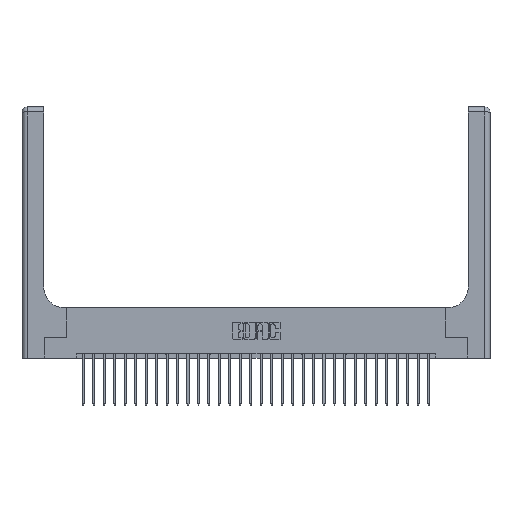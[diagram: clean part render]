
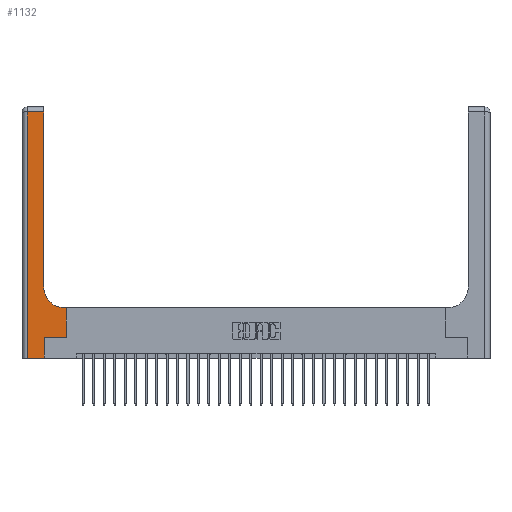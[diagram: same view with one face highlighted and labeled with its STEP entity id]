
A CAD part, top view. The second image highlights one B-rep face of the part: STEP entity #1132.
In plain terms, the highlighted planar face has unit normal (0, 0, 1).
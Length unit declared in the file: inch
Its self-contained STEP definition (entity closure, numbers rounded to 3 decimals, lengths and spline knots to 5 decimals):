
#255 = CARTESIAN_POINT ( 'NONE',  ( 0., 2.94, 0.37 ) ) ;
#324 = VERTEX_POINT ( 'NONE', #21119 ) ;
#370 = EDGE_CURVE ( 'NONE', #13079, #14114, #17188, .T. ) ;
#445 = CARTESIAN_POINT ( 'NONE',  ( 0.06, 2.94, 0.37 ) ) ;
#696 = DIRECTION ( 'NONE',  ( 1., 0., 0. ) ) ;
#823 = VECTOR ( 'NONE', #24106, 39.37008 ) ;
#900 = CARTESIAN_POINT ( 'NONE',  ( 0.51, 0.6, 0.37 ) ) ;
#977 = DIRECTION ( 'NONE',  ( 0., 0., -1. ) ) ;
#1132 = ADVANCED_FACE ( 'NONE', ( #25584 ), #14462, .F. ) ;
#1382 = CARTESIAN_POINT ( 'NONE',  ( 0.06, 3., 0.37 ) ) ;
#1668 = ORIENTED_EDGE ( 'NONE', *, *, #2427, .T. ) ;
#1694 = VECTOR ( 'NONE', #6319, 39.37008 ) ;
#2341 = VERTEX_POINT ( 'NONE', #16649 ) ;
#2427 = EDGE_CURVE ( 'NONE', #14114, #2341, #26855, .T. ) ;
#2792 = AXIS2_PLACEMENT_3D ( 'NONE', #3505, #9783, #10062 ) ;
#3370 = EDGE_CURVE ( 'NONE', #10723, #13079, #20314, .T. ) ;
#3505 = CARTESIAN_POINT ( 'NONE',  ( 0., 3., 0.37 ) ) ;
#3911 = VERTEX_POINT ( 'NONE', #7093 ) ;
#4220 = DIRECTION ( 'NONE',  ( -1., 0., 0. ) ) ;
#4429 = DIRECTION ( 'NONE',  ( -1., 0., 0. ) ) ;
#5190 = EDGE_LOOP ( 'NONE', ( #10304, #11789, #20292, #1668, #28076, #5467, #26640, #19964, #26289 ) ) ;
#5467 = ORIENTED_EDGE ( 'NONE', *, *, #23238, .T. ) ;
#6319 = DIRECTION ( 'NONE',  ( 0., 1., 0. ) ) ;
#6325 = CIRCLE ( 'NONE', #28309, 0.25 ) ;
#6773 = DIRECTION ( 'NONE',  ( 1., 0., 0. ) ) ;
#7093 = CARTESIAN_POINT ( 'NONE',  ( 0.528, 0.6, 0.37 ) ) ;
#7428 = VECTOR ( 'NONE', #19228, 39.37008 ) ;
#7942 = CARTESIAN_POINT ( 'NONE',  ( 0.06, 0., 0.37 ) ) ;
#9665 = CARTESIAN_POINT ( 'NONE',  ( 0.528, 0.25, 0.37 ) ) ;
#9782 = EDGE_CURVE ( 'NONE', #3911, #20388, #15405, .T. ) ;
#9783 = DIRECTION ( 'NONE',  ( 0., 0., -1. ) ) ;
#10062 = DIRECTION ( 'NONE',  ( -1., 0., 0. ) ) ;
#10273 = EDGE_CURVE ( 'NONE', #22266, #10723, #17554, .T. ) ;
#10304 = ORIENTED_EDGE ( 'NONE', *, *, #10273, .T. ) ;
#10723 = VERTEX_POINT ( 'NONE', #15585 ) ;
#11789 = ORIENTED_EDGE ( 'NONE', *, *, #3370, .T. ) ;
#13079 = VERTEX_POINT ( 'NONE', #445 ) ;
#14051 = LINE ( 'NONE', #9665, #14467 ) ;
#14114 = VERTEX_POINT ( 'NONE', #7942 ) ;
#14462 = PLANE ( 'NONE',  #2792 ) ;
#14467 = VECTOR ( 'NONE', #16123, 39.37008 ) ;
#14915 = EDGE_CURVE ( 'NONE', #2341, #21036, #24018, .T. ) ;
#14975 = CARTESIAN_POINT ( 'NONE',  ( 0.265, 0., 0.37 ) ) ;
#15405 = LINE ( 'NONE', #17775, #23778 ) ;
#15585 = CARTESIAN_POINT ( 'NONE',  ( 0.26, 2.94, 0.37 ) ) ;
#16123 = DIRECTION ( 'NONE',  ( 0., 1., 0. ) ) ;
#16649 = CARTESIAN_POINT ( 'NONE',  ( 0.265, 0., 0.37 ) ) ;
#17188 = LINE ( 'NONE', #1382, #7428 ) ;
#17554 = LINE ( 'NONE', #24390, #823 ) ;
#17669 = CARTESIAN_POINT ( 'NONE',  ( 0.265, 0.25, 0.37 ) ) ;
#17775 = CARTESIAN_POINT ( 'NONE',  ( 0.26, 0.6, 0.37 ) ) ;
#17923 = LINE ( 'NONE', #26833, #26446 ) ;
#19228 = DIRECTION ( 'NONE',  ( 0., -1., 0. ) ) ;
#19543 = CARTESIAN_POINT ( 'NONE',  ( 0.51, 0.85, 0.37 ) ) ;
#19964 = ORIENTED_EDGE ( 'NONE', *, *, #9782, .T. ) ;
#20292 = ORIENTED_EDGE ( 'NONE', *, *, #370, .T. ) ;
#20314 = LINE ( 'NONE', #255, #25885 ) ;
#20388 = VERTEX_POINT ( 'NONE', #900 ) ;
#21036 = VERTEX_POINT ( 'NONE', #17669 ) ;
#21119 = CARTESIAN_POINT ( 'NONE',  ( 0.528, 0.25, 0.37 ) ) ;
#21871 = CARTESIAN_POINT ( 'NONE',  ( 0., 0., 0.37 ) ) ;
#22007 = DIRECTION ( 'NONE',  ( 1., 0., 0. ) ) ;
#22266 = VERTEX_POINT ( 'NONE', #24545 ) ;
#22964 = EDGE_CURVE ( 'NONE', #20388, #22266, #6325, .T. ) ;
#23238 = EDGE_CURVE ( 'NONE', #21036, #324, #17923, .T. ) ;
#23778 = VECTOR ( 'NONE', #4429, 39.37008 ) ;
#23899 = VECTOR ( 'NONE', #22007, 39.37008 ) ;
#24018 = LINE ( 'NONE', #14975, #1694 ) ;
#24106 = DIRECTION ( 'NONE',  ( 0., 1., 0. ) ) ;
#24390 = CARTESIAN_POINT ( 'NONE',  ( 0.26, 3., 0.37 ) ) ;
#24545 = CARTESIAN_POINT ( 'NONE',  ( 0.26, 0.85, 0.37 ) ) ;
#25584 = FACE_OUTER_BOUND ( 'NONE', #5190, .T. ) ;
#25885 = VECTOR ( 'NONE', #4220, 39.37008 ) ;
#26289 = ORIENTED_EDGE ( 'NONE', *, *, #22964, .T. ) ;
#26446 = VECTOR ( 'NONE', #6773, 39.37008 ) ;
#26640 = ORIENTED_EDGE ( 'NONE', *, *, #28804, .T. ) ;
#26833 = CARTESIAN_POINT ( 'NONE',  ( 0.265, 0.25, 0.37 ) ) ;
#26855 = LINE ( 'NONE', #21871, #23899 ) ;
#28076 = ORIENTED_EDGE ( 'NONE', *, *, #14915, .T. ) ;
#28309 = AXIS2_PLACEMENT_3D ( 'NONE', #19543, #977, #696 ) ;
#28804 = EDGE_CURVE ( 'NONE', #324, #3911, #14051, .T. ) ;
